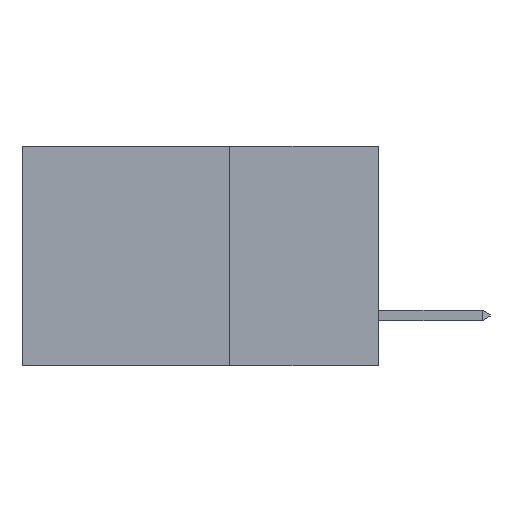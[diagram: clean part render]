
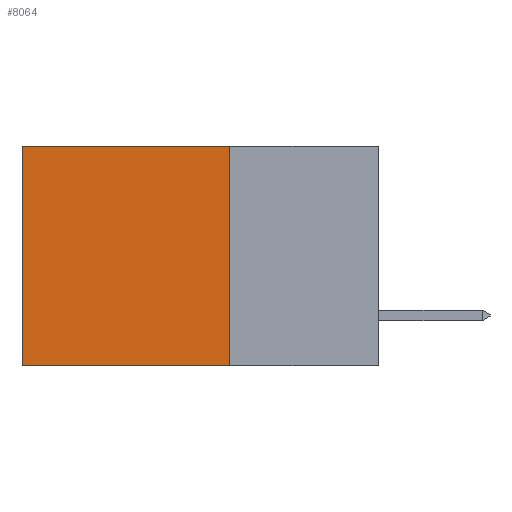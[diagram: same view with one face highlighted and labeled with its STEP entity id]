
A CAD part, left-side view. The second image highlights one B-rep face of the part: STEP entity #8064.
In plain terms, the highlighted planar face has unit normal (-1, 0, 0).
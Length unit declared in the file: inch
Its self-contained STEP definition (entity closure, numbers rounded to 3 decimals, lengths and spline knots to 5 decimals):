
#346 = ORIENTED_EDGE ( 'NONE', *, *, #10614, .T. ) ;
#1111 = ORIENTED_EDGE ( 'NONE', *, *, #9505, .F. ) ;
#1591 = CARTESIAN_POINT ( 'NONE',  ( 0.2615, 0.25, 0. ) ) ;
#1780 = EDGE_CURVE ( 'NONE', #14277, #16362, #4467, .T. ) ;
#2154 = DIRECTION ( 'NONE',  ( 0., 1., 0. ) ) ;
#2435 = CARTESIAN_POINT ( 'NONE',  ( 0.2615, 0.6, -0.37 ) ) ;
#4467 = LINE ( 'NONE', #14871, #8119 ) ;
#4610 = CARTESIAN_POINT ( 'NONE',  ( 0.2615, 0.6, 0. ) ) ;
#4880 = ORIENTED_EDGE ( 'NONE', *, *, #18173, .T. ) ;
#5099 = CARTESIAN_POINT ( 'NONE',  ( 0.2615, 0.25, 0. ) ) ;
#5100 = DIRECTION ( 'NONE',  ( 0., 0., -1. ) ) ;
#5217 = VECTOR ( 'NONE', #13893, 39.37008 ) ;
#5354 = DIRECTION ( 'NONE',  ( 1., 0., 0. ) ) ;
#5455 = CARTESIAN_POINT ( 'NONE',  ( 0.2615, 0.25, -0.37 ) ) ;
#5925 = PLANE ( 'NONE',  #8249 ) ;
#6489 = CARTESIAN_POINT ( 'NONE',  ( 0.2615, 0.25, -0.37 ) ) ;
#6878 = DIRECTION ( 'NONE',  ( 0., 0., -1. ) ) ;
#7341 = LINE ( 'NONE', #5099, #19275 ) ;
#7408 = VECTOR ( 'NONE', #6878, 39.37008 ) ;
#8064 = ADVANCED_FACE ( 'NONE', ( #12434 ), #5925, .F. ) ;
#8119 = VECTOR ( 'NONE', #15333, 39.37008 ) ;
#8249 = AXIS2_PLACEMENT_3D ( 'NONE', #5455, #5354, #5100 ) ;
#9505 = EDGE_CURVE ( 'NONE', #12463, #14277, #15797, .T. ) ;
#10614 = EDGE_CURVE ( 'NONE', #15955, #16362, #13562, .T. ) ;
#11740 = CARTESIAN_POINT ( 'NONE',  ( 0.2615, 0.25, -0.37 ) ) ;
#12434 = FACE_OUTER_BOUND ( 'NONE', #12935, .T. ) ;
#12463 = VERTEX_POINT ( 'NONE', #1591 ) ;
#12935 = EDGE_LOOP ( 'NONE', ( #346, #15206, #1111, #4880 ) ) ;
#13562 = LINE ( 'NONE', #13966, #5217 ) ;
#13893 = DIRECTION ( 'NONE',  ( 0., 0., -1. ) ) ;
#13966 = CARTESIAN_POINT ( 'NONE',  ( 0.2615, 0.6, -0.37 ) ) ;
#14277 = VERTEX_POINT ( 'NONE', #11740 ) ;
#14871 = CARTESIAN_POINT ( 'NONE',  ( 0.2615, 0.25, -0.37 ) ) ;
#15206 = ORIENTED_EDGE ( 'NONE', *, *, #1780, .F. ) ;
#15333 = DIRECTION ( 'NONE',  ( 0., 1., 0. ) ) ;
#15797 = LINE ( 'NONE', #6489, #7408 ) ;
#15955 = VERTEX_POINT ( 'NONE', #4610 ) ;
#16362 = VERTEX_POINT ( 'NONE', #2435 ) ;
#18173 = EDGE_CURVE ( 'NONE', #12463, #15955, #7341, .T. ) ;
#19275 = VECTOR ( 'NONE', #2154, 39.37008 ) ;
